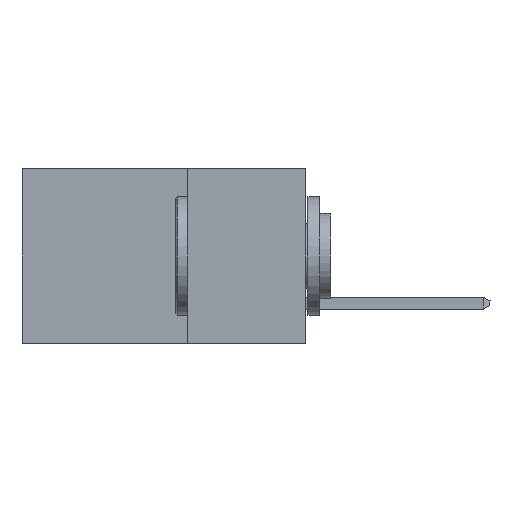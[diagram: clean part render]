
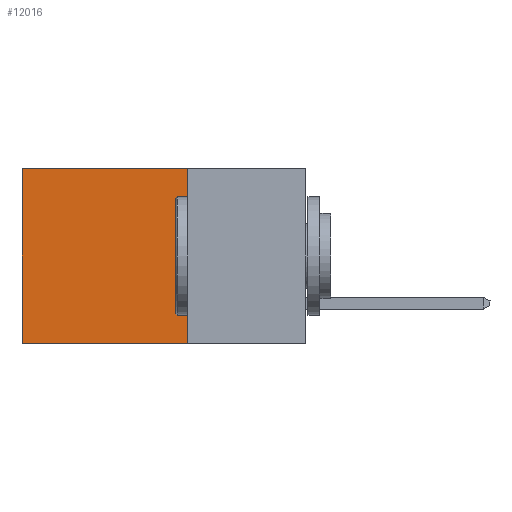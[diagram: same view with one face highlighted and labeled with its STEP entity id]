
A CAD part, left-side view. The second image highlights one B-rep face of the part: STEP entity #12016.
In plain terms, the highlighted planar face has unit normal (-1, 0, 0).
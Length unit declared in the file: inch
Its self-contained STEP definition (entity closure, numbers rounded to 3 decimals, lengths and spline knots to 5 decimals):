
#27 = CARTESIAN_POINT ( 'NONE',  ( 0.298, 0.25, -0.37 ) ) ;
#172 = DIRECTION ( 'NONE',  ( 0., 0., -1. ) ) ;
#912 = DIRECTION ( 'NONE',  ( 0., 1., 0. ) ) ;
#2020 = VERTEX_POINT ( 'NONE', #27 ) ;
#3779 = EDGE_LOOP ( 'NONE', ( #30156, #12754, #8317, #15212 ) ) ;
#4361 = LINE ( 'NONE', #29282, #9904 ) ;
#5135 = LINE ( 'NONE', #28389, #30311 ) ;
#5174 = EDGE_CURVE ( 'NONE', #2020, #11812, #4361, .T. ) ;
#5569 = DIRECTION ( 'NONE',  ( 0., 1., 0. ) ) ;
#7221 = EDGE_CURVE ( 'NONE', #28145, #18902, #28227, .T. ) ;
#8317 = ORIENTED_EDGE ( 'NONE', *, *, #21245, .F. ) ;
#9050 = FACE_OUTER_BOUND ( 'NONE', #3779, .T. ) ;
#9904 = VECTOR ( 'NONE', #912, 39.37008 ) ;
#10120 = AXIS2_PLACEMENT_3D ( 'NONE', #28588, #14360, #172 ) ;
#10920 = CARTESIAN_POINT ( 'NONE',  ( 0.298, 0.25, 0. ) ) ;
#11117 = DIRECTION ( 'NONE',  ( 0., 0., -1. ) ) ;
#11812 = VERTEX_POINT ( 'NONE', #20687 ) ;
#12016 = ADVANCED_FACE ( 'NONE', ( #9050 ), #21477, .F. ) ;
#12754 = ORIENTED_EDGE ( 'NONE', *, *, #5174, .F. ) ;
#14360 = DIRECTION ( 'NONE',  ( 1., 0., 0. ) ) ;
#15212 = ORIENTED_EDGE ( 'NONE', *, *, #7221, .T. ) ;
#15343 = EDGE_CURVE ( 'NONE', #18902, #11812, #5135, .T. ) ;
#15427 = CARTESIAN_POINT ( 'NONE',  ( 0.298, 0.6, 0. ) ) ;
#17357 = CARTESIAN_POINT ( 'NONE',  ( 0.298, 0.25, 0. ) ) ;
#18902 = VERTEX_POINT ( 'NONE', #15427 ) ;
#20687 = CARTESIAN_POINT ( 'NONE',  ( 0.298, 0.6, -0.37 ) ) ;
#21245 = EDGE_CURVE ( 'NONE', #28145, #2020, #26142, .T. ) ;
#21268 = DIRECTION ( 'NONE',  ( 0., 0., -1. ) ) ;
#21477 = PLANE ( 'NONE',  #10120 ) ;
#22978 = CARTESIAN_POINT ( 'NONE',  ( 0.298, 0.25, 0. ) ) ;
#24671 = VECTOR ( 'NONE', #11117, 39.37008 ) ;
#26142 = LINE ( 'NONE', #22978, #24671 ) ;
#27496 = VECTOR ( 'NONE', #5569, 39.37008 ) ;
#28145 = VERTEX_POINT ( 'NONE', #10920 ) ;
#28227 = LINE ( 'NONE', #17357, #27496 ) ;
#28389 = CARTESIAN_POINT ( 'NONE',  ( 0.298, 0.6, 0. ) ) ;
#28588 = CARTESIAN_POINT ( 'NONE',  ( 0.298, 0.25, 0. ) ) ;
#29282 = CARTESIAN_POINT ( 'NONE',  ( 0.298, 0.25, -0.37 ) ) ;
#30156 = ORIENTED_EDGE ( 'NONE', *, *, #15343, .T. ) ;
#30311 = VECTOR ( 'NONE', #21268, 39.37008 ) ;
